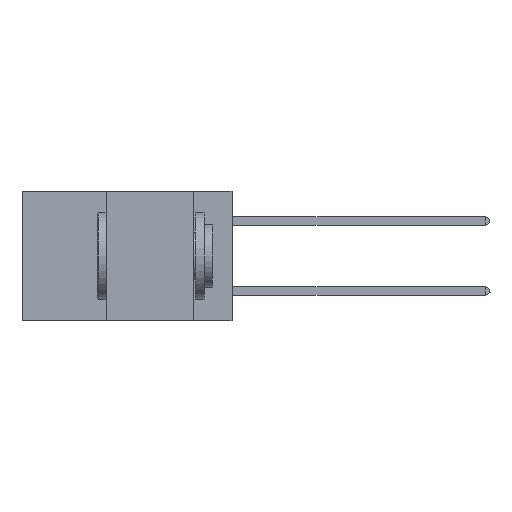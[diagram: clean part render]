
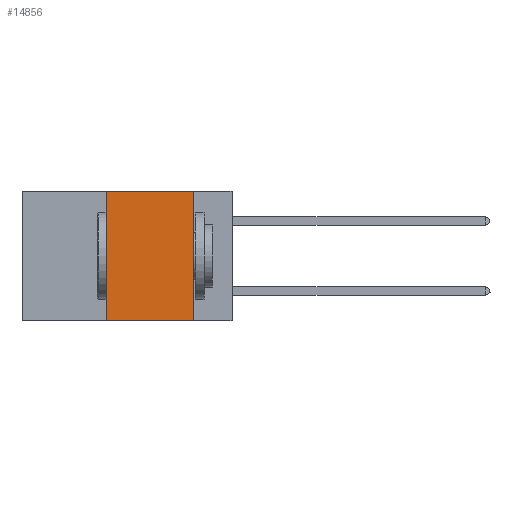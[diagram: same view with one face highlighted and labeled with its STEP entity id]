
A CAD part, left-side view. The second image highlights one B-rep face of the part: STEP entity #14856.
In plain terms, the highlighted planar face has unit normal (-1, 0, 0).
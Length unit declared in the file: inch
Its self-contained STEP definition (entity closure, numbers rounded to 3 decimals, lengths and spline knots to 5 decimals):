
#250 = ORIENTED_EDGE ( 'NONE', *, *, #5557, .F. ) ;
#786 = VERTEX_POINT ( 'NONE', #12204 ) ;
#1590 = AXIS2_PLACEMENT_3D ( 'NONE', #6423, #13897, #3614 ) ;
#1782 = DIRECTION ( 'NONE',  ( 0., 0., -1. ) ) ;
#2198 = DIRECTION ( 'NONE',  ( 0., -1., 0. ) ) ;
#3022 = EDGE_CURVE ( 'NONE', #786, #19181, #10126, .T. ) ;
#3614 = DIRECTION ( 'NONE',  ( 0., 0., -1. ) ) ;
#3640 = VERTEX_POINT ( 'NONE', #9425 ) ;
#3910 = LINE ( 'NONE', #5192, #11372 ) ;
#4346 = ORIENTED_EDGE ( 'NONE', *, *, #6106, .F. ) ;
#5192 = CARTESIAN_POINT ( 'NONE',  ( 0., 0.36, 0. ) ) ;
#5557 = EDGE_CURVE ( 'NONE', #3640, #18703, #14043, .T. ) ;
#6106 = EDGE_CURVE ( 'NONE', #786, #3640, #3910, .T. ) ;
#6423 = CARTESIAN_POINT ( 'NONE',  ( 0., 0.6, 0. ) ) ;
#8157 = DIRECTION ( 'NONE',  ( 0., -1., 0. ) ) ;
#9130 = CARTESIAN_POINT ( 'NONE',  ( 0., 0.11, 0. ) ) ;
#9260 = LINE ( 'NONE', #9130, #15847 ) ;
#9425 = CARTESIAN_POINT ( 'NONE',  ( 0., 0.36, 0. ) ) ;
#9752 = FACE_OUTER_BOUND ( 'NONE', #10290, .T. ) ;
#10126 = LINE ( 'NONE', #17002, #14143 ) ;
#10290 = EDGE_LOOP ( 'NONE', ( #18922, #250, #4346, #11864 ) ) ;
#10963 = VECTOR ( 'NONE', #8157, 39.37008 ) ;
#11372 = VECTOR ( 'NONE', #18507, 39.37008 ) ;
#11535 = CARTESIAN_POINT ( 'NONE',  ( 0., 0.11, 0. ) ) ;
#11864 = ORIENTED_EDGE ( 'NONE', *, *, #3022, .T. ) ;
#12072 = EDGE_CURVE ( 'NONE', #18703, #19181, #9260, .T. ) ;
#12204 = CARTESIAN_POINT ( 'NONE',  ( 0., 0.36, -0.37 ) ) ;
#12592 = CARTESIAN_POINT ( 'NONE',  ( 0., 0.6, 0. ) ) ;
#13897 = DIRECTION ( 'NONE',  ( 1., 0., 0. ) ) ;
#14043 = LINE ( 'NONE', #12592, #10963 ) ;
#14143 = VECTOR ( 'NONE', #2198, 39.37008 ) ;
#14856 = ADVANCED_FACE ( 'NONE', ( #9752 ), #16952, .F. ) ;
#15847 = VECTOR ( 'NONE', #1782, 39.37008 ) ;
#16952 = PLANE ( 'NONE',  #1590 ) ;
#17002 = CARTESIAN_POINT ( 'NONE',  ( 0., 0.6, -0.37 ) ) ;
#18507 = DIRECTION ( 'NONE',  ( 0., 0., 1. ) ) ;
#18703 = VERTEX_POINT ( 'NONE', #11535 ) ;
#18922 = ORIENTED_EDGE ( 'NONE', *, *, #12072, .F. ) ;
#18978 = CARTESIAN_POINT ( 'NONE',  ( 0., 0.11, -0.37 ) ) ;
#19181 = VERTEX_POINT ( 'NONE', #18978 ) ;
